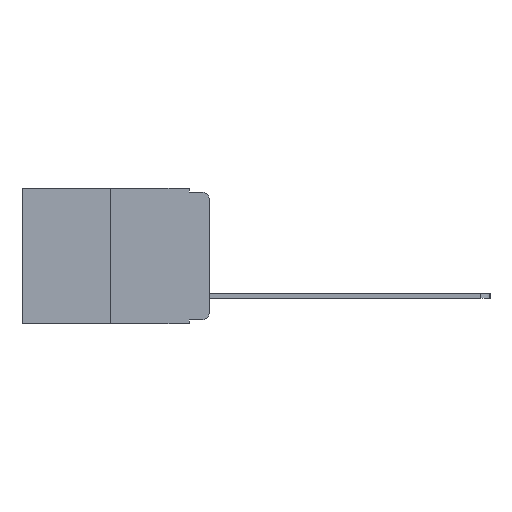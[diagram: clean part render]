
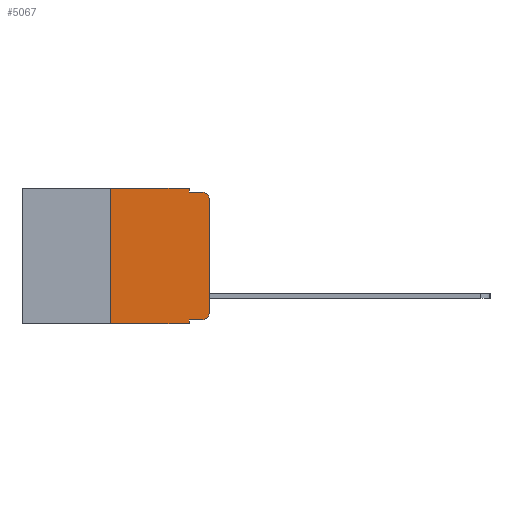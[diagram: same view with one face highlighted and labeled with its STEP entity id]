
A CAD part, left-side view. The second image highlights one B-rep face of the part: STEP entity #5067.
In plain terms, the highlighted planar face has unit normal (-1, 0, 0).
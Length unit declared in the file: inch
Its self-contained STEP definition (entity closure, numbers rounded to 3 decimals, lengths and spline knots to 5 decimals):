
#99 = ORIENTED_EDGE ( 'NONE', *, *, #10685, .T. ) ;
#284 = ORIENTED_EDGE ( 'NONE', *, *, #2503, .T. ) ;
#480 = EDGE_CURVE ( 'NONE', #9231, #17261, #1688, .T. ) ;
#605 = LINE ( 'NONE', #9307, #3902 ) ;
#831 = DIRECTION ( 'NONE',  ( 0., -1., 0. ) ) ;
#1128 = CARTESIAN_POINT ( 'NONE',  ( 0., 0.051, -0.01 ) ) ;
#1169 = ORIENTED_EDGE ( 'NONE', *, *, #7311, .F. ) ;
#1189 = DIRECTION ( 'NONE',  ( 0., -1., 0. ) ) ;
#1604 = DIRECTION ( 'NONE',  ( 1., 0., 0. ) ) ;
#1688 = LINE ( 'NONE', #13646, #9253 ) ;
#2203 = CARTESIAN_POINT ( 'NONE',  ( 0., 0.25, -0.343 ) ) ;
#2219 = ORIENTED_EDGE ( 'NONE', *, *, #7895, .F. ) ;
#2273 = ORIENTED_EDGE ( 'NONE', *, *, #8038, .F. ) ;
#2366 = VECTOR ( 'NONE', #5684, 39.37008 ) ;
#2503 = EDGE_CURVE ( 'NONE', #12133, #5425, #4269, .T. ) ;
#2546 = CIRCLE ( 'NONE', #3977, 0.02 ) ;
#2828 = DIRECTION ( 'NONE',  ( 0., -1., 0. ) ) ;
#2991 = DIRECTION ( 'NONE',  ( 0., 0., 1. ) ) ;
#3023 = VECTOR ( 'NONE', #2828, 39.37008 ) ;
#3523 = VECTOR ( 'NONE', #1189, 39.37008 ) ;
#3569 = CARTESIAN_POINT ( 'NONE',  ( 0., 0.02, -0.313 ) ) ;
#3763 = VERTEX_POINT ( 'NONE', #6001 ) ;
#3902 = VECTOR ( 'NONE', #831, 39.37008 ) ;
#3977 = AXIS2_PLACEMENT_3D ( 'NONE', #3569, #13291, #5022 ) ;
#4269 = CIRCLE ( 'NONE', #7623, 0.02 ) ;
#4330 = VERTEX_POINT ( 'NONE', #2203 ) ;
#4858 = VERTEX_POINT ( 'NONE', #13895 ) ;
#5022 = DIRECTION ( 'NONE',  ( 0., 0., -1. ) ) ;
#5067 = ADVANCED_FACE ( 'NONE', ( #11092 ), #10985, .F. ) ;
#5425 = VERTEX_POINT ( 'NONE', #16037 ) ;
#5684 = DIRECTION ( 'NONE',  ( 0., 0., -1. ) ) ;
#6001 = CARTESIAN_POINT ( 'NONE',  ( 0., 0.051, -0.01 ) ) ;
#6189 = LINE ( 'NONE', #15278, #2366 ) ;
#6753 = CARTESIAN_POINT ( 'NONE',  ( 0., 0.25, 0. ) ) ;
#6863 = VERTEX_POINT ( 'NONE', #16876 ) ;
#7099 = CARTESIAN_POINT ( 'NONE',  ( 0., 0., -0.313 ) ) ;
#7159 = ORIENTED_EDGE ( 'NONE', *, *, #9592, .F. ) ;
#7311 = EDGE_CURVE ( 'NONE', #3763, #5425, #11011, .T. ) ;
#7467 = LINE ( 'NONE', #7972, #10754 ) ;
#7623 = AXIS2_PLACEMENT_3D ( 'NONE', #13140, #13211, #13378 ) ;
#7895 = EDGE_CURVE ( 'NONE', #4330, #9231, #12044, .T. ) ;
#7972 = CARTESIAN_POINT ( 'NONE',  ( 0., 0.051, 0. ) ) ;
#8038 = EDGE_CURVE ( 'NONE', #17261, #3763, #6189, .T. ) ;
#8187 = CARTESIAN_POINT ( 'NONE',  ( 0., 0.473, 0. ) ) ;
#8381 = VECTOR ( 'NONE', #14995, 39.37008 ) ;
#9231 = VERTEX_POINT ( 'NONE', #13999 ) ;
#9247 = EDGE_CURVE ( 'NONE', #10623, #12133, #12408, .T. ) ;
#9253 = VECTOR ( 'NONE', #15824, 39.37008 ) ;
#9307 = CARTESIAN_POINT ( 'NONE',  ( 0., 0.051, -0.333 ) ) ;
#9592 = EDGE_CURVE ( 'NONE', #6863, #9665, #7467, .T. ) ;
#9665 = VERTEX_POINT ( 'NONE', #17517 ) ;
#10150 = CARTESIAN_POINT ( 'NONE',  ( 0., 0.051, 0. ) ) ;
#10623 = VERTEX_POINT ( 'NONE', #7099 ) ;
#10685 = EDGE_CURVE ( 'NONE', #4330, #9665, #17216, .T. ) ;
#10754 = VECTOR ( 'NONE', #12070, 39.37008 ) ;
#10985 = PLANE ( 'NONE',  #17584 ) ;
#11011 = LINE ( 'NONE', #1128, #3523 ) ;
#11092 = FACE_OUTER_BOUND ( 'NONE', #11316, .T. ) ;
#11297 = ORIENTED_EDGE ( 'NONE', *, *, #11479, .T. ) ;
#11316 = EDGE_LOOP ( 'NONE', ( #13133, #284, #1169, #2273, #11957, #2219, #99, #7159, #11297, #17023 ) ) ;
#11435 = CARTESIAN_POINT ( 'NONE',  ( 0., 0., 0. ) ) ;
#11446 = DIRECTION ( 'NONE',  ( 0., 0., -1. ) ) ;
#11479 = EDGE_CURVE ( 'NONE', #6863, #4858, #605, .T. ) ;
#11957 = ORIENTED_EDGE ( 'NONE', *, *, #480, .F. ) ;
#12044 = LINE ( 'NONE', #6753, #8381 ) ;
#12070 = DIRECTION ( 'NONE',  ( 0., 0., -1. ) ) ;
#12133 = VERTEX_POINT ( 'NONE', #14817 ) ;
#12408 = LINE ( 'NONE', #11435, #15969 ) ;
#13133 = ORIENTED_EDGE ( 'NONE', *, *, #9247, .T. ) ;
#13140 = CARTESIAN_POINT ( 'NONE',  ( 0., 0.02, -0.03 ) ) ;
#13211 = DIRECTION ( 'NONE',  ( -1., 0., 0. ) ) ;
#13291 = DIRECTION ( 'NONE',  ( -1., 0., 0. ) ) ;
#13378 = DIRECTION ( 'NONE',  ( 0., 0., -1. ) ) ;
#13646 = CARTESIAN_POINT ( 'NONE',  ( 0., 0.473, 0. ) ) ;
#13895 = CARTESIAN_POINT ( 'NONE',  ( 0., 0.02, -0.333 ) ) ;
#13999 = CARTESIAN_POINT ( 'NONE',  ( 0., 0.25, 0. ) ) ;
#14817 = CARTESIAN_POINT ( 'NONE',  ( 0., 0., -0.03 ) ) ;
#14995 = DIRECTION ( 'NONE',  ( 0., 0., 1. ) ) ;
#15278 = CARTESIAN_POINT ( 'NONE',  ( 0., 0.051, 0. ) ) ;
#15383 = CARTESIAN_POINT ( 'NONE',  ( 0., 0.473, -0.343 ) ) ;
#15728 = EDGE_CURVE ( 'NONE', #4858, #10623, #2546, .T. ) ;
#15824 = DIRECTION ( 'NONE',  ( 0., -1., 0. ) ) ;
#15969 = VECTOR ( 'NONE', #2991, 39.37008 ) ;
#16037 = CARTESIAN_POINT ( 'NONE',  ( 0., 0.02, -0.01 ) ) ;
#16876 = CARTESIAN_POINT ( 'NONE',  ( 0., 0.051, -0.333 ) ) ;
#17023 = ORIENTED_EDGE ( 'NONE', *, *, #15728, .T. ) ;
#17216 = LINE ( 'NONE', #15383, #3023 ) ;
#17261 = VERTEX_POINT ( 'NONE', #10150 ) ;
#17517 = CARTESIAN_POINT ( 'NONE',  ( 0., 0.051, -0.343 ) ) ;
#17584 = AXIS2_PLACEMENT_3D ( 'NONE', #8187, #1604, #11446 ) ;
